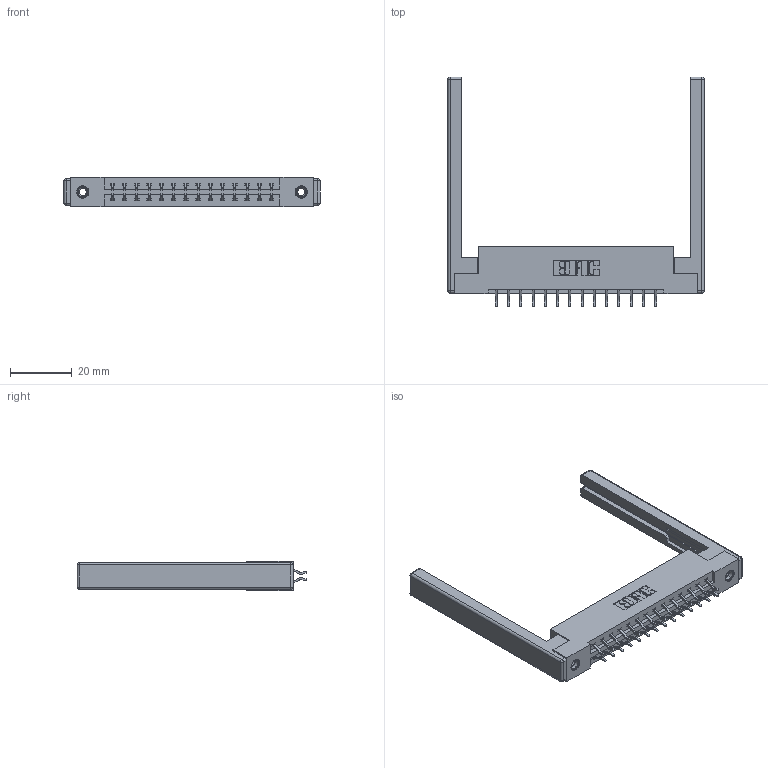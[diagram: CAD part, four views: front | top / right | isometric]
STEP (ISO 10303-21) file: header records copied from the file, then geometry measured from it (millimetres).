
FILE_DESCRIPTION (( 'STEP AP203' ), '1' );
FILE_NAME ('337-028-556-268.STEP', '2019-10-08T17:20:10', ( '' ), ( '' ), 'SwSTEP 2.0', 'SolidWorks 2016', '' );
FILE_SCHEMA (( 'CONFIG_CONTROL_DESIGN' ));
Length unit declared in the file: inch
Products named in the file (5): 337-028-556-268; 345-292-001_556 Tail; 307-220-068; 345-250-001_345-250-001-102; 337 Part_Flush Mounting Lugs - 0.156 Dia-TI
Assembly tree (33 placements, depth 2):
  337-028-556-268
    337 Part_Flush Mounting Lugs - 0.156 Dia-TI
    345-292-001_556 Tail  x28
    345-250-001_345-250-001-102  x2
    307-220-068  x2
Bounding box: 82.91 x 74.31 x 9.4 mm (x, y, z)
Volume: 12748.2 mm3; surface area: 13187.7 mm2
Topology: 33 solids, 33 shells, 1948 faces, 5713 edges, 3750 vertices
Faces by surface type: plane 1334, cylinder 590, cone 12, sphere 8, torus 4
Entity records: 17456 total; most frequent: CARTESIAN_POINT 2943, ORIENTED_EDGE 2856, DIRECTION 2614, EDGE_CURVE 1428, LINE 1242, VECTOR 1242, VERTEX_POINT 942, AXIS2_PLACEMENT_3D 686
